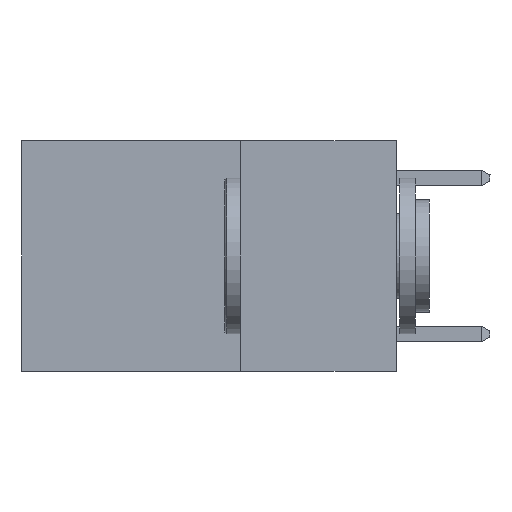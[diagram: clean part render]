
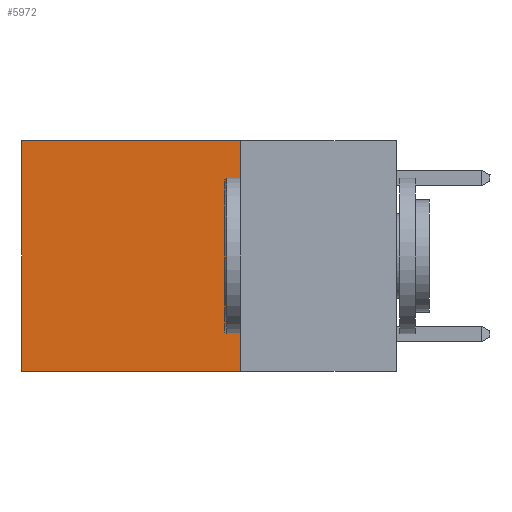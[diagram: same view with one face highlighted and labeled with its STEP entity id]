
A CAD part, left-side view. The second image highlights one B-rep face of the part: STEP entity #5972.
In plain terms, the highlighted planar face has unit normal (-1, 0, 0).
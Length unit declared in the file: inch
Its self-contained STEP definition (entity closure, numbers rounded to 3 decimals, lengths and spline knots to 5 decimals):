
#502 = ORIENTED_EDGE ( 'NONE', *, *, #1493, .T. ) ;
#875 = CARTESIAN_POINT ( 'NONE',  ( 0.2625, 0.25, 0. ) ) ;
#920 = CARTESIAN_POINT ( 'NONE',  ( 0.2625, 0.25, 0. ) ) ;
#1042 = LINE ( 'NONE', #4152, #6702 ) ;
#1112 = EDGE_CURVE ( 'NONE', #1903, #2503, #7756, .T. ) ;
#1276 = ORIENTED_EDGE ( 'NONE', *, *, #2737, .F. ) ;
#1493 = EDGE_CURVE ( 'NONE', #1903, #9610, #1517, .T. ) ;
#1517 = LINE ( 'NONE', #875, #5882 ) ;
#1609 = PLANE ( 'NONE',  #6235 ) ;
#1657 = DIRECTION ( 'NONE',  ( 0., 1., 0. ) ) ;
#1811 = CARTESIAN_POINT ( 'NONE',  ( 0.2625, 0.6, -0.37 ) ) ;
#1876 = DIRECTION ( 'NONE',  ( 0., 0., -1. ) ) ;
#1903 = VERTEX_POINT ( 'NONE', #3886 ) ;
#2503 = VERTEX_POINT ( 'NONE', #4327 ) ;
#2737 = EDGE_CURVE ( 'NONE', #2503, #6174, #4942, .T. ) ;
#2909 = ORIENTED_EDGE ( 'NONE', *, *, #5181, .T. ) ;
#3101 = CARTESIAN_POINT ( 'NONE',  ( 0.2625, 0.25, -0.37 ) ) ;
#3886 = CARTESIAN_POINT ( 'NONE',  ( 0.2625, 0.25, 0. ) ) ;
#4152 = CARTESIAN_POINT ( 'NONE',  ( 0.2625, 0.6, 0. ) ) ;
#4327 = CARTESIAN_POINT ( 'NONE',  ( 0.2625, 0.25, -0.37 ) ) ;
#4942 = LINE ( 'NONE', #3101, #7104 ) ;
#5015 = VECTOR ( 'NONE', #5285, 39.37008 ) ;
#5181 = EDGE_CURVE ( 'NONE', #9610, #6174, #1042, .T. ) ;
#5285 = DIRECTION ( 'NONE',  ( 0., 0., -1. ) ) ;
#5882 = VECTOR ( 'NONE', #1657, 39.37008 ) ;
#5972 = ADVANCED_FACE ( 'NONE', ( #8823 ), #1609, .F. ) ;
#6174 = VERTEX_POINT ( 'NONE', #1811 ) ;
#6235 = AXIS2_PLACEMENT_3D ( 'NONE', #920, #6368, #8927 ) ;
#6368 = DIRECTION ( 'NONE',  ( 1., 0., 0. ) ) ;
#6554 = CARTESIAN_POINT ( 'NONE',  ( 0.2625, 0.6, 0. ) ) ;
#6702 = VECTOR ( 'NONE', #1876, 39.37008 ) ;
#6920 = CARTESIAN_POINT ( 'NONE',  ( 0.2625, 0.25, 0. ) ) ;
#7104 = VECTOR ( 'NONE', #10356, 39.37008 ) ;
#7756 = LINE ( 'NONE', #6920, #5015 ) ;
#7844 = EDGE_LOOP ( 'NONE', ( #2909, #1276, #10262, #502 ) ) ;
#8823 = FACE_OUTER_BOUND ( 'NONE', #7844, .T. ) ;
#8927 = DIRECTION ( 'NONE',  ( 0., 0., -1. ) ) ;
#9610 = VERTEX_POINT ( 'NONE', #6554 ) ;
#10262 = ORIENTED_EDGE ( 'NONE', *, *, #1112, .F. ) ;
#10356 = DIRECTION ( 'NONE',  ( 0., 1., 0. ) ) ;
